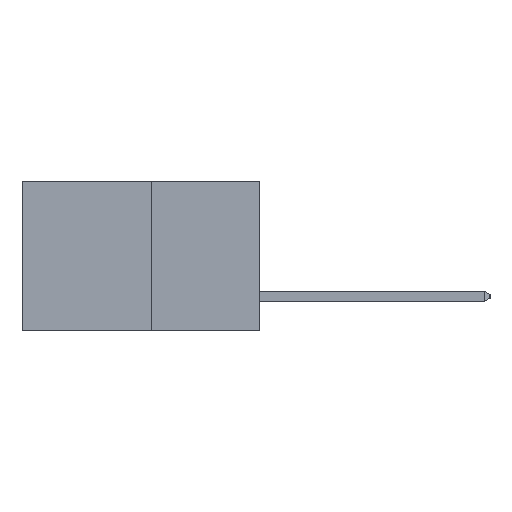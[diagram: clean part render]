
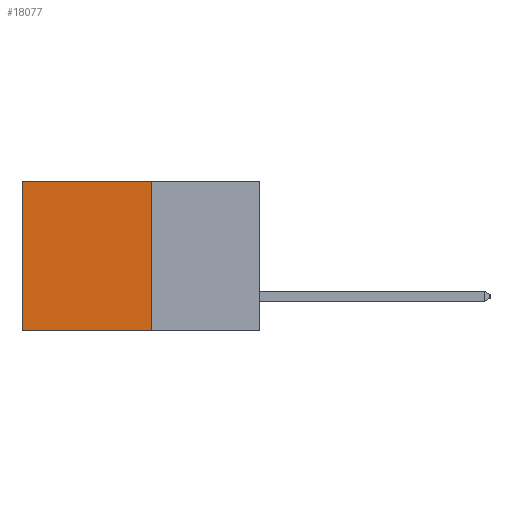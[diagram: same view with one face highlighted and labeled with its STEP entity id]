
A CAD part, left-side view. The second image highlights one B-rep face of the part: STEP entity #18077.
In plain terms, the highlighted planar face has unit normal (-1, 0, 0).
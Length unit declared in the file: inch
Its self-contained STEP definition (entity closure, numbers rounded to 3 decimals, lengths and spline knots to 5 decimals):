
#221 = DIRECTION ( 'NONE',  ( 0., 0., -1. ) ) ;
#348 = CARTESIAN_POINT ( 'NONE',  ( 0.277, 0.59, -0.37 ) ) ;
#957 = VERTEX_POINT ( 'NONE', #24277 ) ;
#1344 = LINE ( 'NONE', #29545, #19593 ) ;
#2610 = ORIENTED_EDGE ( 'NONE', *, *, #28503, .T. ) ;
#3351 = CARTESIAN_POINT ( 'NONE',  ( 0.277, 0.27, 0. ) ) ;
#3400 = VERTEX_POINT ( 'NONE', #348 ) ;
#3792 = CARTESIAN_POINT ( 'NONE',  ( 0.277, 0.27, 0. ) ) ;
#3938 = LINE ( 'NONE', #3792, #15907 ) ;
#7666 = EDGE_LOOP ( 'NONE', ( #18593, #26561, #30244, #2610 ) ) ;
#7848 = VERTEX_POINT ( 'NONE', #22180 ) ;
#8579 = DIRECTION ( 'NONE',  ( 0., 1., 0. ) ) ;
#9257 = DIRECTION ( 'NONE',  ( 0., 1., 0. ) ) ;
#11720 = LINE ( 'NONE', #14287, #24299 ) ;
#13829 = EDGE_CURVE ( 'NONE', #17682, #957, #11720, .T. ) ;
#14287 = CARTESIAN_POINT ( 'NONE',  ( 0.277, 0.27, -0.37 ) ) ;
#14529 = DIRECTION ( 'NONE',  ( 1., 0., 0. ) ) ;
#15907 = VECTOR ( 'NONE', #8579, 39.37008 ) ;
#17682 = VERTEX_POINT ( 'NONE', #3351 ) ;
#17934 = DIRECTION ( 'NONE',  ( 0., 0., -1. ) ) ;
#17994 = VECTOR ( 'NONE', #9257, 39.37008 ) ;
#18077 = ADVANCED_FACE ( 'NONE', ( #19266 ), #26224, .F. ) ;
#18593 = ORIENTED_EDGE ( 'NONE', *, *, #23448, .T. ) ;
#19266 = FACE_OUTER_BOUND ( 'NONE', #7666, .T. ) ;
#19593 = VECTOR ( 'NONE', #17934, 39.37008 ) ;
#20245 = LINE ( 'NONE', #30476, #17994 ) ;
#21030 = DIRECTION ( 'NONE',  ( 0., 0., -1. ) ) ;
#22180 = CARTESIAN_POINT ( 'NONE',  ( 0.277, 0.59, 0. ) ) ;
#23448 = EDGE_CURVE ( 'NONE', #7848, #3400, #1344, .T. ) ;
#24277 = CARTESIAN_POINT ( 'NONE',  ( 0.277, 0.27, -0.37 ) ) ;
#24299 = VECTOR ( 'NONE', #21030, 39.37008 ) ;
#26224 = PLANE ( 'NONE',  #28182 ) ;
#26561 = ORIENTED_EDGE ( 'NONE', *, *, #29248, .F. ) ;
#28182 = AXIS2_PLACEMENT_3D ( 'NONE', #28555, #14529, #221 ) ;
#28503 = EDGE_CURVE ( 'NONE', #17682, #7848, #3938, .T. ) ;
#28555 = CARTESIAN_POINT ( 'NONE',  ( 0.277, 0.27, -0.37 ) ) ;
#29248 = EDGE_CURVE ( 'NONE', #957, #3400, #20245, .T. ) ;
#29545 = CARTESIAN_POINT ( 'NONE',  ( 0.277, 0.59, -0.37 ) ) ;
#30244 = ORIENTED_EDGE ( 'NONE', *, *, #13829, .F. ) ;
#30476 = CARTESIAN_POINT ( 'NONE',  ( 0.277, 0.27, -0.37 ) ) ;
